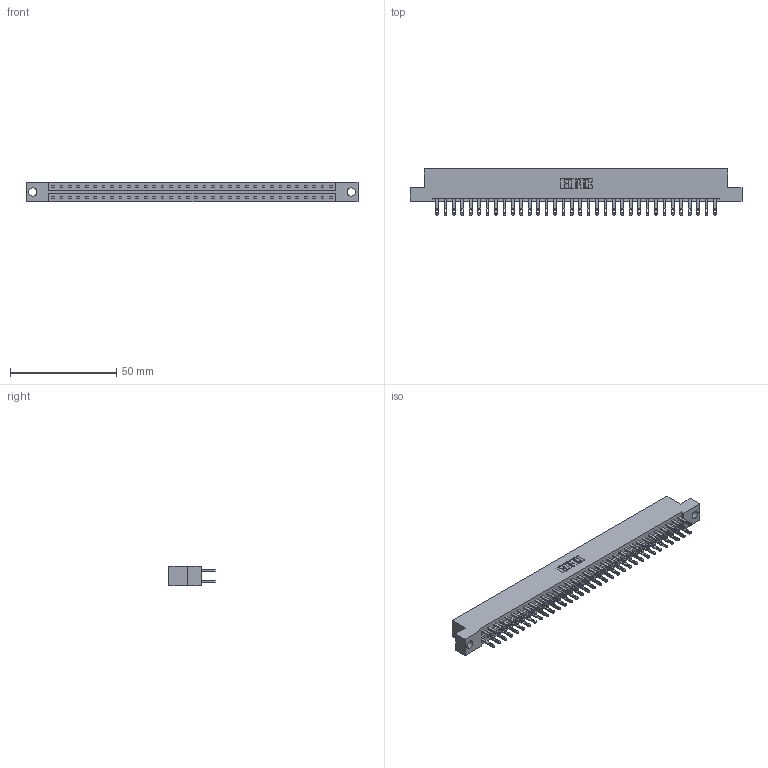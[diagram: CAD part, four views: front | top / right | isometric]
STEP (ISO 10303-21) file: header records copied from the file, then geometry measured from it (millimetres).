
FILE_DESCRIPTION (( 'STEP AP203' ), '1' );
FILE_NAME ('833-068-500-204.STEP', '2020-06-05T09:56:58', ( '' ), ( '' ), 'SwSTEP 2.0', 'SolidWorks 2020', '' );
FILE_SCHEMA (( 'CONFIG_CONTROL_DESIGN' ));
Length unit declared in the file: inch
Products named in the file (3): 345-292-001_345-293-100; 833-068-500-204; 833 Part_Flush - .156 Dia - TH
Assembly tree (69 placements, depth 2):
  833-068-500-204
    833 Part_Flush - .156 Dia - TH
    345-292-001_345-293-100  x68
Bounding box: 156.26 x 21.85 x 9.4 mm (x, y, z)
Volume: 15998.5 mm3; surface area: 19375.9 mm2
Topology: 69 solids, 69 shells, 3378 faces, 10307 edges, 6870 vertices
Faces by surface type: plane 2110, cylinder 1268
Entity records: 22841 total; most frequent: CARTESIAN_POINT 3794, ORIENTED_EDGE 3730, DIRECTION 3257, EDGE_CURVE 1865, LINE 1733, VECTOR 1733, VERTEX_POINT 1242, AXIS2_PLACEMENT_3D 762
